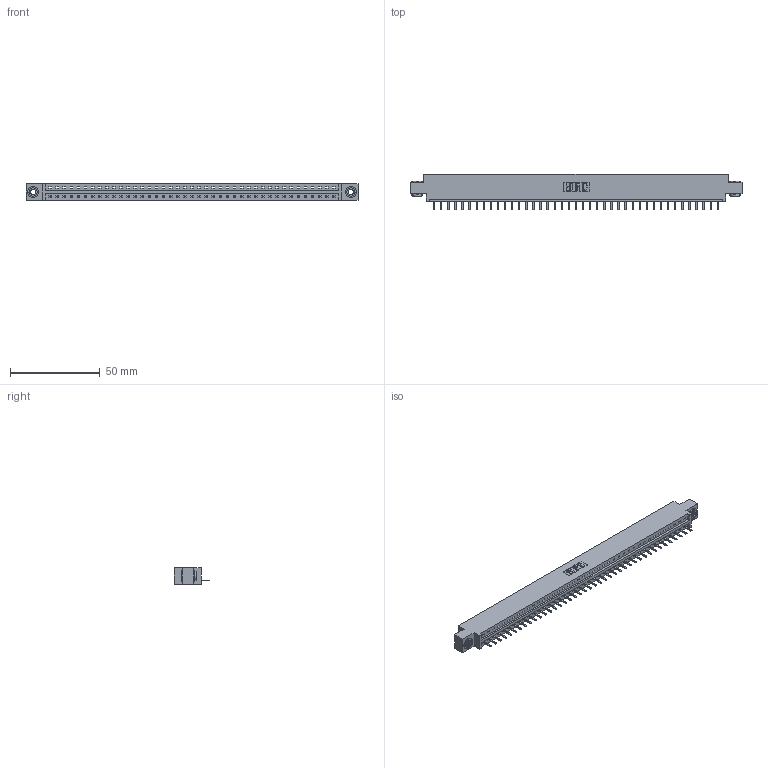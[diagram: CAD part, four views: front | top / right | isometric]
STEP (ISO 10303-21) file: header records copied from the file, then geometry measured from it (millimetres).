
FILE_DESCRIPTION (( 'STEP AP203' ), '1' );
FILE_NAME ('337-041-520-603.STEP', '2019-10-01T20:24:31', ( '' ), ( '' ), 'SwSTEP 2.0', 'SolidWorks 2016', '' );
FILE_SCHEMA (( 'CONFIG_CONTROL_DESIGN' ));
Length unit declared in the file: inch
Products named in the file (4): 345-250-002_345-250-002-102; 337-041-520-603; 337 Part_0.170 Offset - 0.156 Dia-TH; 345-292-001_345-293-120
Assembly tree (44 placements, depth 2):
  337-041-520-603
    337 Part_0.170 Offset - 0.156 Dia-TH
    345-292-001_345-293-120  x41
    345-250-002_345-250-002-102  x2
Bounding box: 185.47 x 20.02 x 9.4 mm (x, y, z)
Volume: 19048 mm3; surface area: 19582.4 mm2
Topology: 44 solids, 44 shells, 2862 faces, 8435 edges, 5510 vertices
Faces by surface type: plane 2052, cylinder 802, cone 8
Entity records: 31502 total; most frequent: CARTESIAN_POINT 5476, ORIENTED_EDGE 5434, DIRECTION 4633, EDGE_CURVE 2717, VECTOR 2561, LINE 2561, VERTEX_POINT 1806, AXIS2_PLACEMENT_3D 1036
